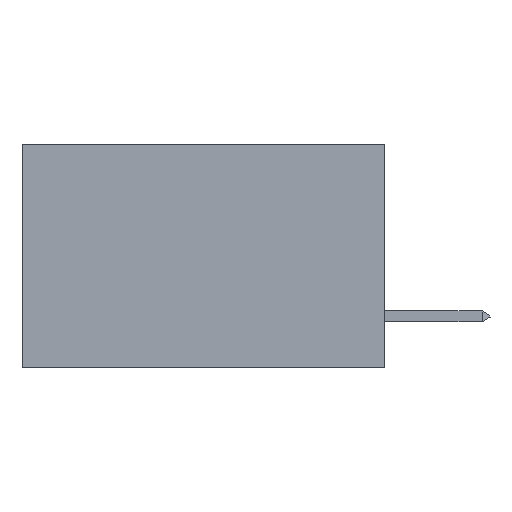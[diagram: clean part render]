
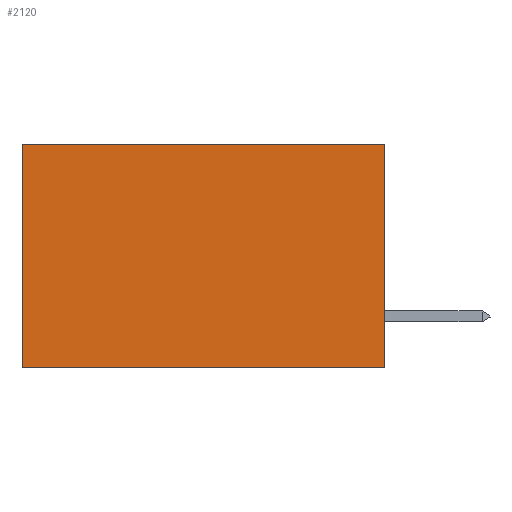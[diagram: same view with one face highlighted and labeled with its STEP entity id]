
A CAD part, left-side view. The second image highlights one B-rep face of the part: STEP entity #2120.
In plain terms, the highlighted planar face has unit normal (-1, 0, 0).
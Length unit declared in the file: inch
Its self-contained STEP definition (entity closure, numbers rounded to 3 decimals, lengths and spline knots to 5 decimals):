
#204 = FACE_OUTER_BOUND ( 'NONE', #15641, .T. ) ;
#296 = LINE ( 'NONE', #4365, #14000 ) ;
#869 = ORIENTED_EDGE ( 'NONE', *, *, #3484, .T. ) ;
#1233 = DIRECTION ( 'NONE',  ( 0., 0., -1. ) ) ;
#1312 = VERTEX_POINT ( 'NONE', #6565 ) ;
#2120 = ADVANCED_FACE ( 'NONE', ( #204 ), #6078, .F. ) ;
#2243 = CARTESIAN_POINT ( 'NONE',  ( 0.2875, 0., 0. ) ) ;
#2420 = VERTEX_POINT ( 'NONE', #16486 ) ;
#3484 = EDGE_CURVE ( 'NONE', #9992, #1312, #5519, .T. ) ;
#4230 = VERTEX_POINT ( 'NONE', #2243 ) ;
#4326 = DIRECTION ( 'NONE',  ( 1., 0., 0. ) ) ;
#4365 = CARTESIAN_POINT ( 'NONE',  ( 0.2875, 0., 0. ) ) ;
#4718 = DIRECTION ( 'NONE',  ( 0., 1., 0. ) ) ;
#5399 = EDGE_CURVE ( 'NONE', #4230, #2420, #296, .T. ) ;
#5519 = LINE ( 'NONE', #15058, #11581 ) ;
#6078 = PLANE ( 'NONE',  #10810 ) ;
#6565 = CARTESIAN_POINT ( 'NONE',  ( 0.2875, 0.6, -0.37 ) ) ;
#7094 = DIRECTION ( 'NONE',  ( 0., 1., 0. ) ) ;
#7312 = VECTOR ( 'NONE', #4718, 39.37008 ) ;
#7947 = LINE ( 'NONE', #11357, #7312 ) ;
#9269 = CARTESIAN_POINT ( 'NONE',  ( 0.2875, 0.6, 0. ) ) ;
#9593 = EDGE_CURVE ( 'NONE', #2420, #1312, #10971, .T. ) ;
#9948 = CARTESIAN_POINT ( 'NONE',  ( 0.2875, 0., -0.37 ) ) ;
#9992 = VERTEX_POINT ( 'NONE', #9269 ) ;
#10810 = AXIS2_PLACEMENT_3D ( 'NONE', #13567, #4326, #1233 ) ;
#10971 = LINE ( 'NONE', #9948, #16602 ) ;
#11357 = CARTESIAN_POINT ( 'NONE',  ( 0.2875, 0., 0. ) ) ;
#11581 = VECTOR ( 'NONE', #12156, 39.37008 ) ;
#12156 = DIRECTION ( 'NONE',  ( 0., 0., -1. ) ) ;
#13567 = CARTESIAN_POINT ( 'NONE',  ( 0.2875, 0., 0. ) ) ;
#14000 = VECTOR ( 'NONE', #16589, 39.37008 ) ;
#14100 = ORIENTED_EDGE ( 'NONE', *, *, #5399, .F. ) ;
#14613 = ORIENTED_EDGE ( 'NONE', *, *, #9593, .F. ) ;
#14999 = EDGE_CURVE ( 'NONE', #4230, #9992, #7947, .T. ) ;
#15058 = CARTESIAN_POINT ( 'NONE',  ( 0.2875, 0.6, 0. ) ) ;
#15641 = EDGE_LOOP ( 'NONE', ( #869, #14613, #14100, #15884 ) ) ;
#15884 = ORIENTED_EDGE ( 'NONE', *, *, #14999, .T. ) ;
#16486 = CARTESIAN_POINT ( 'NONE',  ( 0.2875, 0., -0.37 ) ) ;
#16589 = DIRECTION ( 'NONE',  ( 0., 0., -1. ) ) ;
#16602 = VECTOR ( 'NONE', #7094, 39.37008 ) ;
